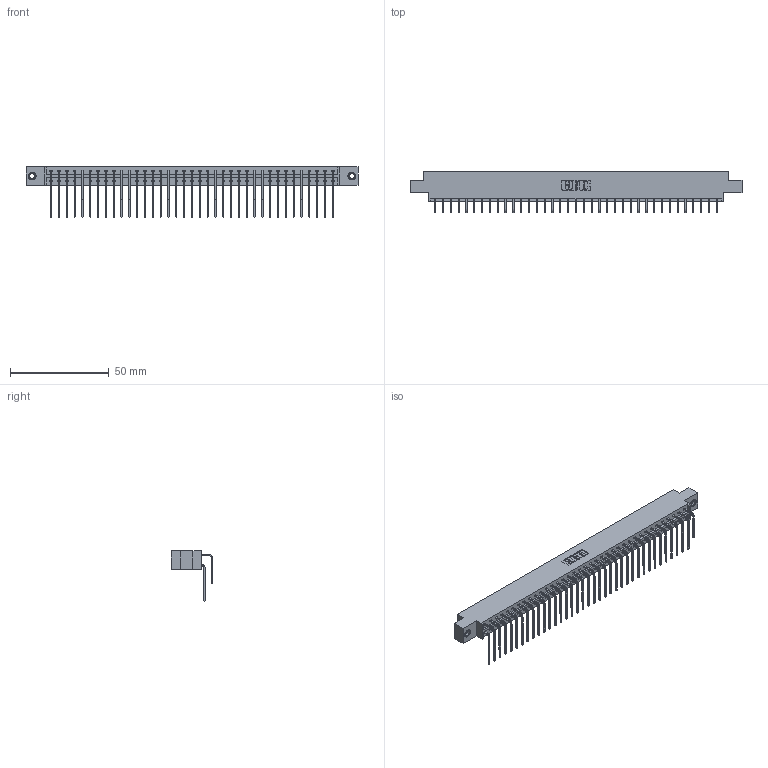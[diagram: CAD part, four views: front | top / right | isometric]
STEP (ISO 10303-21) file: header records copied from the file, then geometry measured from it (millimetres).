
FILE_DESCRIPTION (( 'STEP AP203' ), '1' );
FILE_NAME ('833-074-559-807.STEP', '2020-06-05T17:32:02', ( '' ), ( '' ), 'SwSTEP 2.0', 'SolidWorks 2020', '' );
FILE_SCHEMA (( 'CONFIG_CONTROL_DESIGN' ));
Length unit declared in the file: inch
Products named in the file (5): 833-074-559-807; 833 Part_Offset - .156 Dia - TI; 345-292-001_559 Tail - 2; 345-250-001_345-250-005-103; 345-292-001_558 559 Tail - 1
Assembly tree (77 placements, depth 2):
  833-074-559-807
    833 Part_Offset - .156 Dia - TI
    345-292-001_558 559 Tail - 1  x37
    345-292-001_559 Tail - 2  x37
    345-250-001_345-250-005-103  x2
Bounding box: 168.15 x 20.9 x 25.53 mm (x, y, z)
Volume: 17305.8 mm3; surface area: 22787.3 mm2
Topology: 77 solids, 77 shells, 4174 faces, 12373 edges, 8142 vertices
Faces by surface type: plane 2918, cylinder 1240, cone 12, torus 4
Entity records: 27552 total; most frequent: CARTESIAN_POINT 4608, ORIENTED_EDGE 4486, DIRECTION 3957, EDGE_CURVE 2243, LINE 2055, VECTOR 2055, VERTEX_POINT 1488, AXIS2_PLACEMENT_3D 951
